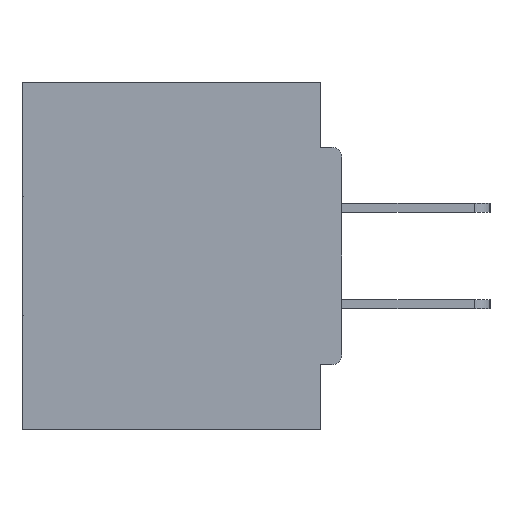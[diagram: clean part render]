
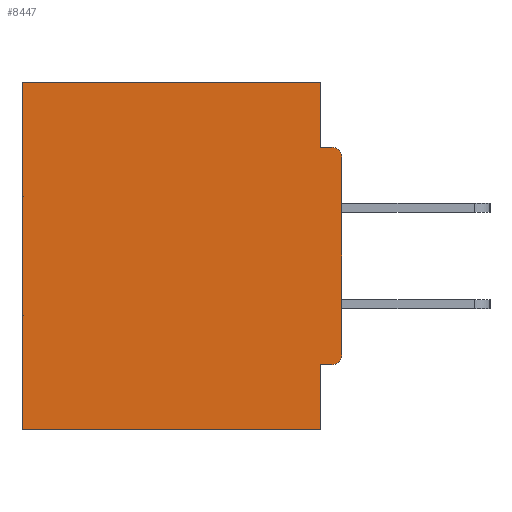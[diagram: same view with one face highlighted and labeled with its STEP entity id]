
A CAD part, left-side view. The second image highlights one B-rep face of the part: STEP entity #8447.
In plain terms, the highlighted planar face has unit normal (-1, 0, 0).
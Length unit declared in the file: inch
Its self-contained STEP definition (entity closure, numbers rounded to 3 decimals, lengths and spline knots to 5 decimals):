
#235 = EDGE_CURVE ( 'NONE', #2154, #24111, #25875, .T. ) ;
#263 = LINE ( 'NONE', #5717, #36582 ) ;
#545 = CARTESIAN_POINT ( 'NONE',  ( 0.298, 0.015, -0.1085 ) ) ;
#1354 = CIRCLE ( 'NONE', #19423, 0.015 ) ;
#1383 = CARTESIAN_POINT ( 'NONE',  ( 0.298, 0.031, -0.5 ) ) ;
#1422 = CARTESIAN_POINT ( 'NONE',  ( 0.298, 0., 0. ) ) ;
#1634 = CARTESIAN_POINT ( 'NONE',  ( 0.298, 0., -0.5 ) ) ;
#2154 = VERTEX_POINT ( 'NONE', #23050 ) ;
#2861 = CARTESIAN_POINT ( 'NONE',  ( 0.298, 0., 0. ) ) ;
#4707 = LINE ( 'NONE', #2861, #30151 ) ;
#5717 = CARTESIAN_POINT ( 'NONE',  ( 0.298, 0.46, 0. ) ) ;
#6363 = ORIENTED_EDGE ( 'NONE', *, *, #235, .T. ) ;
#6521 = LINE ( 'NONE', #19568, #37326 ) ;
#7834 = DIRECTION ( 'NONE',  ( 0., 0., -1. ) ) ;
#8447 = ADVANCED_FACE ( 'NONE', ( #34889 ), #13964, .F. ) ;
#8619 = DIRECTION ( 'NONE',  ( 0., -1., 0. ) ) ;
#9054 = CARTESIAN_POINT ( 'NONE',  ( 0.298, 0.031, -0.5 ) ) ;
#9511 = ORIENTED_EDGE ( 'NONE', *, *, #33130, .F. ) ;
#10233 = EDGE_CURVE ( 'NONE', #2154, #34345, #30533, .T. ) ;
#11308 = EDGE_CURVE ( 'NONE', #19512, #16405, #6521, .T. ) ;
#12107 = CARTESIAN_POINT ( 'NONE',  ( 0.298, 0., -0.0935 ) ) ;
#12427 = DIRECTION ( 'NONE',  ( -1., 0., 0. ) ) ;
#12504 = CARTESIAN_POINT ( 'NONE',  ( 0.298, 0.46, -0.5 ) ) ;
#13964 = PLANE ( 'NONE',  #28079 ) ;
#14872 = DIRECTION ( 'NONE',  ( 0., 1., 0. ) ) ;
#15076 = VECTOR ( 'NONE', #39080, 39.37008 ) ;
#15276 = ORIENTED_EDGE ( 'NONE', *, *, #31770, .T. ) ;
#15651 = DIRECTION ( 'NONE',  ( 0., 0., -1. ) ) ;
#16030 = CARTESIAN_POINT ( 'NONE',  ( 0.298, 0.031, 0. ) ) ;
#16405 = VERTEX_POINT ( 'NONE', #37389 ) ;
#16499 = EDGE_CURVE ( 'NONE', #19512, #24266, #24905, .T. ) ;
#16868 = CARTESIAN_POINT ( 'NONE',  ( 0.298, 0., -0.4065 ) ) ;
#17079 = VECTOR ( 'NONE', #26880, 39.37008 ) ;
#17490 = AXIS2_PLACEMENT_3D ( 'NONE', #25266, #12427, #15651 ) ;
#19423 = AXIS2_PLACEMENT_3D ( 'NONE', #545, #38542, #29402 ) ;
#19512 = VERTEX_POINT ( 'NONE', #16030 ) ;
#19568 = CARTESIAN_POINT ( 'NONE',  ( 0.298, 0., 0. ) ) ;
#19576 = DIRECTION ( 'NONE',  ( 0., 0., -1. ) ) ;
#20188 = VERTEX_POINT ( 'NONE', #40406 ) ;
#20196 = CARTESIAN_POINT ( 'NONE',  ( 0.298, 0.031, -0.5 ) ) ;
#22105 = DIRECTION ( 'NONE',  ( 0., 0., -1. ) ) ;
#22494 = CARTESIAN_POINT ( 'NONE',  ( 0.298, 0., -0.3915 ) ) ;
#22590 = ORIENTED_EDGE ( 'NONE', *, *, #28602, .F. ) ;
#22660 = LINE ( 'NONE', #12107, #38546 ) ;
#22705 = ORIENTED_EDGE ( 'NONE', *, *, #30682, .F. ) ;
#23050 = CARTESIAN_POINT ( 'NONE',  ( 0.298, 0.015, -0.4065 ) ) ;
#24111 = VERTEX_POINT ( 'NONE', #22494 ) ;
#24266 = VERTEX_POINT ( 'NONE', #28100 ) ;
#24905 = LINE ( 'NONE', #9054, #27368 ) ;
#25266 = CARTESIAN_POINT ( 'NONE',  ( 0.298, 0.015, -0.3915 ) ) ;
#25875 = CIRCLE ( 'NONE', #17490, 0.015 ) ;
#25899 = CARTESIAN_POINT ( 'NONE',  ( 0.298, 0.031, -0.4065 ) ) ;
#25900 = LINE ( 'NONE', #1634, #37278 ) ;
#26538 = LINE ( 'NONE', #1383, #17079 ) ;
#26880 = DIRECTION ( 'NONE',  ( 0., 0., -1. ) ) ;
#26912 = DIRECTION ( 'NONE',  ( 1., 0., 0. ) ) ;
#27077 = ORIENTED_EDGE ( 'NONE', *, *, #40710, .T. ) ;
#27368 = VECTOR ( 'NONE', #31457, 39.37008 ) ;
#28079 = AXIS2_PLACEMENT_3D ( 'NONE', #1422, #26912, #7834 ) ;
#28100 = CARTESIAN_POINT ( 'NONE',  ( 0.298, 0.031, -0.0935 ) ) ;
#28602 = EDGE_CURVE ( 'NONE', #34345, #40880, #26538, .T. ) ;
#29402 = DIRECTION ( 'NONE',  ( 0., 0., -1. ) ) ;
#29838 = ORIENTED_EDGE ( 'NONE', *, *, #33337, .F. ) ;
#30151 = VECTOR ( 'NONE', #22105, 39.37008 ) ;
#30415 = ORIENTED_EDGE ( 'NONE', *, *, #16499, .F. ) ;
#30533 = LINE ( 'NONE', #16868, #15076 ) ;
#30682 = EDGE_CURVE ( 'NONE', #40880, #34329, #25900, .T. ) ;
#31122 = VERTEX_POINT ( 'NONE', #39014 ) ;
#31457 = DIRECTION ( 'NONE',  ( 0., 0., -1. ) ) ;
#31770 = EDGE_CURVE ( 'NONE', #20188, #31122, #1354, .T. ) ;
#32018 = ORIENTED_EDGE ( 'NONE', *, *, #10233, .F. ) ;
#33130 = EDGE_CURVE ( 'NONE', #20188, #24111, #4707, .T. ) ;
#33337 = EDGE_CURVE ( 'NONE', #24266, #31122, #22660, .T. ) ;
#34329 = VERTEX_POINT ( 'NONE', #12504 ) ;
#34345 = VERTEX_POINT ( 'NONE', #25899 ) ;
#34889 = FACE_OUTER_BOUND ( 'NONE', #40860, .T. ) ;
#35095 = DIRECTION ( 'NONE',  ( 0., 1., 0. ) ) ;
#35892 = ORIENTED_EDGE ( 'NONE', *, *, #11308, .T. ) ;
#36582 = VECTOR ( 'NONE', #19576, 39.37008 ) ;
#37278 = VECTOR ( 'NONE', #14872, 39.37008 ) ;
#37326 = VECTOR ( 'NONE', #35095, 39.37008 ) ;
#37389 = CARTESIAN_POINT ( 'NONE',  ( 0.298, 0.46, 0. ) ) ;
#38542 = DIRECTION ( 'NONE',  ( -1., 0., 0. ) ) ;
#38546 = VECTOR ( 'NONE', #8619, 39.37008 ) ;
#39014 = CARTESIAN_POINT ( 'NONE',  ( 0.298, 0.015, -0.0935 ) ) ;
#39080 = DIRECTION ( 'NONE',  ( 0., 1., 0. ) ) ;
#40406 = CARTESIAN_POINT ( 'NONE',  ( 0.298, 0., -0.1085 ) ) ;
#40710 = EDGE_CURVE ( 'NONE', #16405, #34329, #263, .T. ) ;
#40860 = EDGE_LOOP ( 'NONE', ( #15276, #29838, #30415, #35892, #27077, #22705, #22590, #32018, #6363, #9511 ) ) ;
#40880 = VERTEX_POINT ( 'NONE', #20196 ) ;
